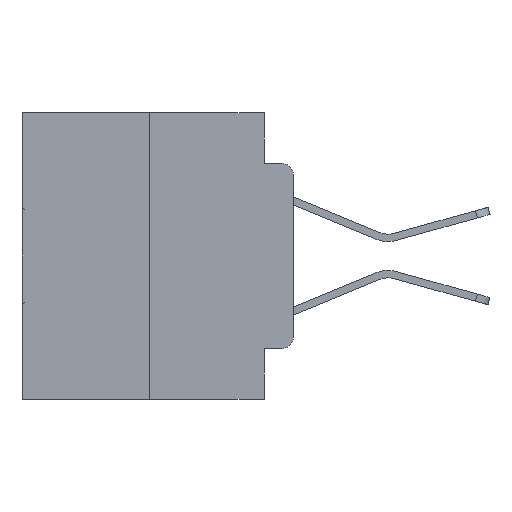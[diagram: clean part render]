
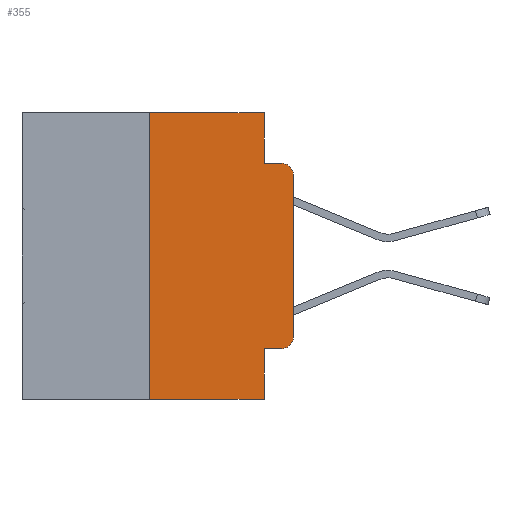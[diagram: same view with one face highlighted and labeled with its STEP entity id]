
A CAD part, left-side view. The second image highlights one B-rep face of the part: STEP entity #355.
In plain terms, the highlighted planar face has unit normal (-1, 0, 0).
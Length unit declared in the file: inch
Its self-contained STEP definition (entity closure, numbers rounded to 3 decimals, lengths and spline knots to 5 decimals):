
#192 = ORIENTED_EDGE ( 'NONE', *, *, #19232, .T. ) ;
#355 = ADVANCED_FACE ( 'NONE', ( #18136 ), #27101, .F. ) ;
#733 = VECTOR ( 'NONE', #9620, 39.37008 ) ;
#983 = DIRECTION ( 'NONE',  ( 0., -1., 0. ) ) ;
#985 = AXIS2_PLACEMENT_3D ( 'NONE', #3424, #3280, #1374 ) ;
#1337 = CARTESIAN_POINT ( 'NONE',  ( 0., 0.051, -0.5 ) ) ;
#1374 = DIRECTION ( 'NONE',  ( 0., 0., -1. ) ) ;
#1639 = VERTEX_POINT ( 'NONE', #7516 ) ;
#2600 = CARTESIAN_POINT ( 'NONE',  ( 0., 0.051, 0. ) ) ;
#2721 = CARTESIAN_POINT ( 'NONE',  ( 0., 0.051, 0. ) ) ;
#3185 = LINE ( 'NONE', #20444, #14712 ) ;
#3280 = DIRECTION ( 'NONE',  ( 1., 0., 0. ) ) ;
#3390 = DIRECTION ( 'NONE',  ( 0., 0., -1. ) ) ;
#3424 = CARTESIAN_POINT ( 'NONE',  ( 0., 0.473, 0. ) ) ;
#3459 = EDGE_LOOP ( 'NONE', ( #3953, #29589, #30084, #8684, #5506, #15708, #192, #19642, #23137, #15305 ) ) ;
#3953 = ORIENTED_EDGE ( 'NONE', *, *, #15604, .T. ) ;
#3959 = LINE ( 'NONE', #5871, #29891 ) ;
#4295 = AXIS2_PLACEMENT_3D ( 'NONE', #24865, #20169, #3390 ) ;
#4388 = DIRECTION ( 'NONE',  ( 0., 0., -1. ) ) ;
#4502 = CARTESIAN_POINT ( 'NONE',  ( 0., 0.02, -0.0885 ) ) ;
#4905 = CARTESIAN_POINT ( 'NONE',  ( 0., 0.051, -0.0885 ) ) ;
#5506 = ORIENTED_EDGE ( 'NONE', *, *, #25705, .F. ) ;
#5871 = CARTESIAN_POINT ( 'NONE',  ( 0., 0.051, -0.4115 ) ) ;
#6148 = EDGE_CURVE ( 'NONE', #22465, #7992, #3185, .T. ) ;
#6891 = CARTESIAN_POINT ( 'NONE',  ( 0., 0.02, -0.3915 ) ) ;
#7516 = CARTESIAN_POINT ( 'NONE',  ( 0., 0., -0.1085 ) ) ;
#7992 = VERTEX_POINT ( 'NONE', #24467 ) ;
#8684 = ORIENTED_EDGE ( 'NONE', *, *, #6148, .F. ) ;
#9270 = DIRECTION ( 'NONE',  ( 0., 0., 1. ) ) ;
#9620 = DIRECTION ( 'NONE',  ( 0., -1., 0. ) ) ;
#9755 = VERTEX_POINT ( 'NONE', #21678 ) ;
#9883 = VECTOR ( 'NONE', #28486, 39.37008 ) ;
#11336 = DIRECTION ( 'NONE',  ( 0., -1., 0. ) ) ;
#11673 = LINE ( 'NONE', #4905, #733 ) ;
#11880 = DIRECTION ( 'NONE',  ( 0., 0., 1. ) ) ;
#12805 = CARTESIAN_POINT ( 'NONE',  ( 0., 0.25, 0. ) ) ;
#13125 = VECTOR ( 'NONE', #9270, 39.37008 ) ;
#13359 = LINE ( 'NONE', #20270, #28214 ) ;
#13842 = VECTOR ( 'NONE', #11880, 39.37008 ) ;
#14232 = VERTEX_POINT ( 'NONE', #1337 ) ;
#14518 = LINE ( 'NONE', #2600, #9883 ) ;
#14712 = VECTOR ( 'NONE', #27334, 39.37008 ) ;
#14724 = EDGE_CURVE ( 'NONE', #22414, #14772, #3959, .T. ) ;
#14772 = VERTEX_POINT ( 'NONE', #27492 ) ;
#15305 = ORIENTED_EDGE ( 'NONE', *, *, #21382, .T. ) ;
#15307 = EDGE_CURVE ( 'NONE', #22414, #14232, #14518, .T. ) ;
#15416 = VERTEX_POINT ( 'NONE', #12805 ) ;
#15602 = VECTOR ( 'NONE', #24640, 39.37008 ) ;
#15604 = EDGE_CURVE ( 'NONE', #9755, #1639, #23782, .T. ) ;
#15708 = ORIENTED_EDGE ( 'NONE', *, *, #19513, .F. ) ;
#16567 = CARTESIAN_POINT ( 'NONE',  ( 0., 0.25, -0.5 ) ) ;
#17035 = EDGE_CURVE ( 'NONE', #1639, #23302, #26312, .T. ) ;
#18136 = FACE_OUTER_BOUND ( 'NONE', #3459, .T. ) ;
#18607 = VERTEX_POINT ( 'NONE', #16567 ) ;
#19232 = EDGE_CURVE ( 'NONE', #18607, #14232, #24494, .T. ) ;
#19513 = EDGE_CURVE ( 'NONE', #18607, #15416, #26181, .T. ) ;
#19642 = ORIENTED_EDGE ( 'NONE', *, *, #15307, .F. ) ;
#20169 = DIRECTION ( 'NONE',  ( -1., 0., 0. ) ) ;
#20270 = CARTESIAN_POINT ( 'NONE',  ( 0., 0.473, 0. ) ) ;
#20444 = CARTESIAN_POINT ( 'NONE',  ( 0., 0.051, 0. ) ) ;
#21189 = CARTESIAN_POINT ( 'NONE',  ( 0., 0.25, 0. ) ) ;
#21248 = AXIS2_PLACEMENT_3D ( 'NONE', #6891, #28201, #4388 ) ;
#21382 = EDGE_CURVE ( 'NONE', #14772, #9755, #22740, .T. ) ;
#21678 = CARTESIAN_POINT ( 'NONE',  ( 0., 0., -0.3915 ) ) ;
#22414 = VERTEX_POINT ( 'NONE', #23902 ) ;
#22465 = VERTEX_POINT ( 'NONE', #2721 ) ;
#22740 = CIRCLE ( 'NONE', #21248, 0.02 ) ;
#23137 = ORIENTED_EDGE ( 'NONE', *, *, #14724, .T. ) ;
#23302 = VERTEX_POINT ( 'NONE', #4502 ) ;
#23782 = LINE ( 'NONE', #26582, #13842 ) ;
#23902 = CARTESIAN_POINT ( 'NONE',  ( 0., 0.051, -0.4115 ) ) ;
#24467 = CARTESIAN_POINT ( 'NONE',  ( 0., 0.051, -0.0885 ) ) ;
#24494 = LINE ( 'NONE', #24804, #15602 ) ;
#24640 = DIRECTION ( 'NONE',  ( 0., -1., 0. ) ) ;
#24804 = CARTESIAN_POINT ( 'NONE',  ( 0., 0.473, -0.5 ) ) ;
#24865 = CARTESIAN_POINT ( 'NONE',  ( 0., 0.02, -0.1085 ) ) ;
#25705 = EDGE_CURVE ( 'NONE', #15416, #22465, #13359, .T. ) ;
#26181 = LINE ( 'NONE', #21189, #13125 ) ;
#26312 = CIRCLE ( 'NONE', #4295, 0.02 ) ;
#26582 = CARTESIAN_POINT ( 'NONE',  ( 0., 0., 0. ) ) ;
#26761 = EDGE_CURVE ( 'NONE', #7992, #23302, #11673, .T. ) ;
#27101 = PLANE ( 'NONE',  #985 ) ;
#27334 = DIRECTION ( 'NONE',  ( 0., 0., -1. ) ) ;
#27492 = CARTESIAN_POINT ( 'NONE',  ( 0., 0.02, -0.4115 ) ) ;
#28201 = DIRECTION ( 'NONE',  ( -1., 0., 0. ) ) ;
#28214 = VECTOR ( 'NONE', #11336, 39.37008 ) ;
#28486 = DIRECTION ( 'NONE',  ( 0., 0., -1. ) ) ;
#29589 = ORIENTED_EDGE ( 'NONE', *, *, #17035, .T. ) ;
#29891 = VECTOR ( 'NONE', #983, 39.37008 ) ;
#30084 = ORIENTED_EDGE ( 'NONE', *, *, #26761, .F. ) ;
